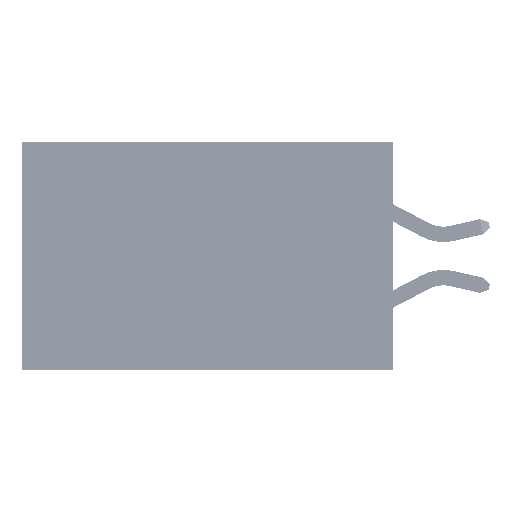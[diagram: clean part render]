
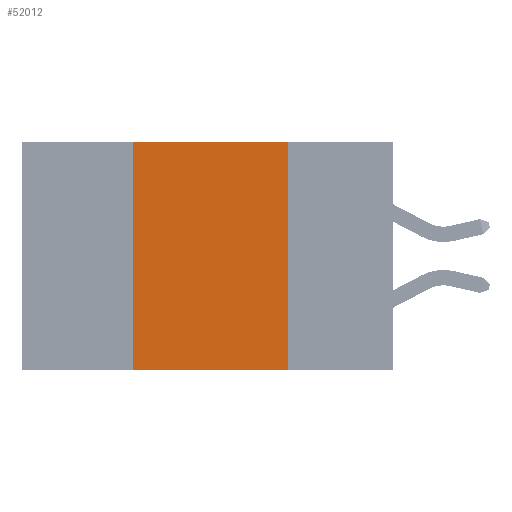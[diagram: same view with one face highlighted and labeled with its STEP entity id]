
A CAD part, left-side view. The second image highlights one B-rep face of the part: STEP entity #52012.
In plain terms, the highlighted planar face has unit normal (-1, 0, 0).
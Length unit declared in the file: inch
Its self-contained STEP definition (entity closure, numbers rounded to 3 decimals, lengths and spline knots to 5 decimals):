
#78 = EDGE_LOOP ( 'NONE', ( #7011, #22253, #14663, #1507 ) ) ;
#472 = DIRECTION ( 'NONE',  ( 0., -1., 0. ) ) ;
#1507 = ORIENTED_EDGE ( 'NONE', *, *, #46569, .T. ) ;
#2653 = CARTESIAN_POINT ( 'NONE',  ( 0., 0.6, 0. ) ) ;
#3935 = CARTESIAN_POINT ( 'NONE',  ( 0., 0.17, 0. ) ) ;
#5904 = DIRECTION ( 'NONE',  ( 1., 0., 0. ) ) ;
#7011 = ORIENTED_EDGE ( 'NONE', *, *, #38300, .F. ) ;
#7962 = VERTEX_POINT ( 'NONE', #19108 ) ;
#9949 = CARTESIAN_POINT ( 'NONE',  ( 0., 0.6, 0. ) ) ;
#14005 = PLANE ( 'NONE',  #30827 ) ;
#14663 = ORIENTED_EDGE ( 'NONE', *, *, #43654, .F. ) ;
#16127 = CARTESIAN_POINT ( 'NONE',  ( 0., 0.42, 0. ) ) ;
#17138 = LINE ( 'NONE', #3935, #47490 ) ;
#19108 = CARTESIAN_POINT ( 'NONE',  ( 0., 0.17, -0.37 ) ) ;
#19111 = DIRECTION ( 'NONE',  ( 0., -1., 0. ) ) ;
#22253 = ORIENTED_EDGE ( 'NONE', *, *, #36443, .F. ) ;
#26172 = FACE_OUTER_BOUND ( 'NONE', #78, .T. ) ;
#29772 = CARTESIAN_POINT ( 'NONE',  ( 0., 0.17, 0. ) ) ;
#30827 = AXIS2_PLACEMENT_3D ( 'NONE', #9949, #5904, #30994 ) ;
#30994 = DIRECTION ( 'NONE',  ( 0., 0., -1. ) ) ;
#31429 = VERTEX_POINT ( 'NONE', #16127 ) ;
#32522 = LINE ( 'NONE', #40331, #49609 ) ;
#32804 = DIRECTION ( 'NONE',  ( 0., 0., -1. ) ) ;
#35910 = VECTOR ( 'NONE', #472, 39.37008 ) ;
#36111 = VERTEX_POINT ( 'NONE', #38013 ) ;
#36443 = EDGE_CURVE ( 'NONE', #31429, #49443, #39603, .T. ) ;
#37436 = CARTESIAN_POINT ( 'NONE',  ( 0., 0.6, -0.37 ) ) ;
#38013 = CARTESIAN_POINT ( 'NONE',  ( 0., 0.42, -0.37 ) ) ;
#38300 = EDGE_CURVE ( 'NONE', #49443, #7962, #17138, .T. ) ;
#39603 = LINE ( 'NONE', #2653, #40631 ) ;
#40331 = CARTESIAN_POINT ( 'NONE',  ( 0., 0.42, 0. ) ) ;
#40631 = VECTOR ( 'NONE', #19111, 39.37008 ) ;
#43654 = EDGE_CURVE ( 'NONE', #36111, #31429, #32522, .T. ) ;
#46569 = EDGE_CURVE ( 'NONE', #36111, #7962, #49546, .T. ) ;
#47490 = VECTOR ( 'NONE', #32804, 39.37008 ) ;
#48403 = DIRECTION ( 'NONE',  ( 0., 0., 1. ) ) ;
#49443 = VERTEX_POINT ( 'NONE', #29772 ) ;
#49546 = LINE ( 'NONE', #37436, #35910 ) ;
#49609 = VECTOR ( 'NONE', #48403, 39.37008 ) ;
#52012 = ADVANCED_FACE ( 'NONE', ( #26172 ), #14005, .F. ) ;
